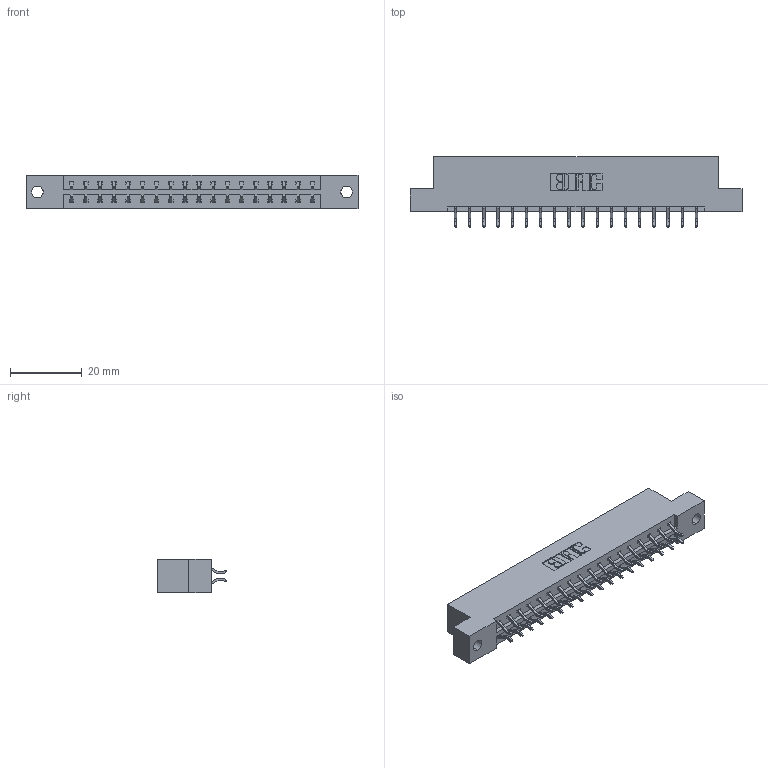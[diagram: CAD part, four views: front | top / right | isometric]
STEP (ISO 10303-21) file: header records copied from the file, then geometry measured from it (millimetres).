
FILE_DESCRIPTION (( 'STEP AP203' ), '1' );
FILE_NAME ('333-036-556-202.STEP', '2018-08-03T01:35:34', ( '' ), ( '' ), 'SwSTEP 2.0', 'SolidWorks 2016', '' );
FILE_SCHEMA (( 'CONFIG_CONTROL_DESIGN' ));
Length unit declared in the file: inch
Products named in the file (3): 333 Part_Flush - .128 Dia; 345-292-001_556 Tail; 333-036-556-202
Assembly tree (37 placements, depth 2):
  333-036-556-202
    333 Part_Flush - .128 Dia
    345-292-001_556 Tail  x36
Bounding box: 92.86 x 19.57 x 9.4 mm (x, y, z)
Volume: 9218.2 mm3; surface area: 10331.4 mm2
Topology: 37 solids, 37 shells, 2202 faces, 6539 edges, 4310 vertices
Faces by surface type: plane 1510, cylinder 692
Entity records: 14907 total; most frequent: CARTESIAN_POINT 2514, ORIENTED_EDGE 2438, DIRECTION 2179, EDGE_CURVE 1219, VECTOR 1083, LINE 1083, VERTEX_POINT 810, AXIS2_PLACEMENT_3D 548
